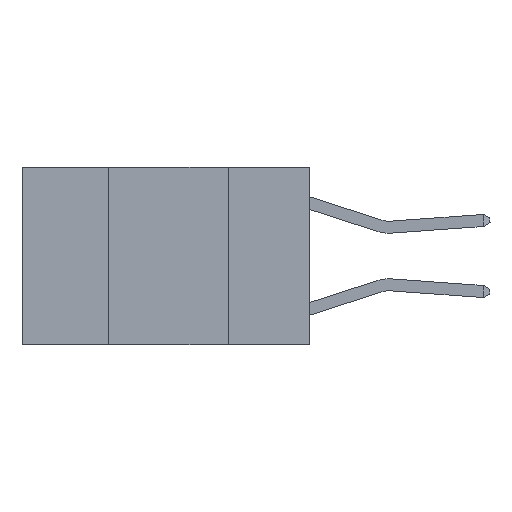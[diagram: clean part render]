
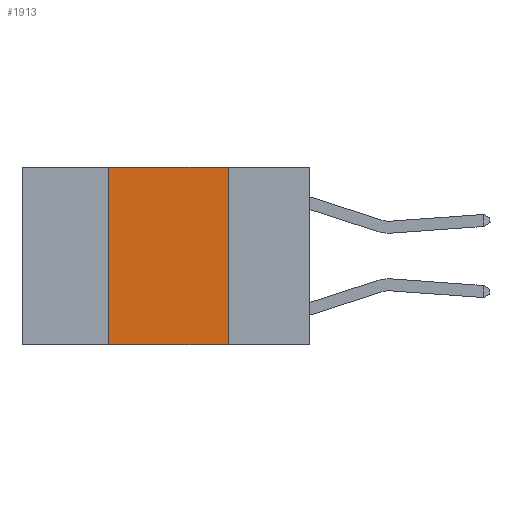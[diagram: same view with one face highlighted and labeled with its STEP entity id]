
A CAD part, left-side view. The second image highlights one B-rep face of the part: STEP entity #1913.
In plain terms, the highlighted planar face has unit normal (-1, 0, 0).
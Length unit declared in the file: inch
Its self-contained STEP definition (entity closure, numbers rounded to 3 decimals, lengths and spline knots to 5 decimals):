
#260 = VECTOR ( 'NONE', #7534, 39.37008 ) ;
#488 = CARTESIAN_POINT ( 'NONE',  ( 0., 0.17, -0.37 ) ) ;
#896 = CARTESIAN_POINT ( 'NONE',  ( 0., 0.6, -0.37 ) ) ;
#914 = LINE ( 'NONE', #11250, #3595 ) ;
#1346 = AXIS2_PLACEMENT_3D ( 'NONE', #8076, #11667, #6297 ) ;
#1599 = VERTEX_POINT ( 'NONE', #488 ) ;
#1626 = ORIENTED_EDGE ( 'NONE', *, *, #5721, .F. ) ;
#1913 = ADVANCED_FACE ( 'NONE', ( #11395 ), #10786, .F. ) ;
#2496 = CARTESIAN_POINT ( 'NONE',  ( 0., 0.6, 0. ) ) ;
#3595 = VECTOR ( 'NONE', #9520, 39.37008 ) ;
#3722 = VERTEX_POINT ( 'NONE', #9327 ) ;
#3993 = VERTEX_POINT ( 'NONE', #6340 ) ;
#4448 = VECTOR ( 'NONE', #7520, 39.37008 ) ;
#4730 = CARTESIAN_POINT ( 'NONE',  ( 0., 0.42, 0. ) ) ;
#4772 = LINE ( 'NONE', #2496, #11710 ) ;
#4922 = ORIENTED_EDGE ( 'NONE', *, *, #9820, .T. ) ;
#5017 = VERTEX_POINT ( 'NONE', #7310 ) ;
#5721 = EDGE_CURVE ( 'NONE', #5017, #3722, #4772, .T. ) ;
#6297 = DIRECTION ( 'NONE',  ( 0., 0., -1. ) ) ;
#6340 = CARTESIAN_POINT ( 'NONE',  ( 0., 0.42, -0.37 ) ) ;
#6675 = ORIENTED_EDGE ( 'NONE', *, *, #8371, .F. ) ;
#7098 = DIRECTION ( 'NONE',  ( 0., -1., 0. ) ) ;
#7310 = CARTESIAN_POINT ( 'NONE',  ( 0., 0.42, 0. ) ) ;
#7520 = DIRECTION ( 'NONE',  ( 0., 0., 1. ) ) ;
#7534 = DIRECTION ( 'NONE',  ( 0., -1., 0. ) ) ;
#8076 = CARTESIAN_POINT ( 'NONE',  ( 0., 0.6, 0. ) ) ;
#8241 = EDGE_CURVE ( 'NONE', #3993, #5017, #11684, .T. ) ;
#8371 = EDGE_CURVE ( 'NONE', #3722, #1599, #914, .T. ) ;
#9327 = CARTESIAN_POINT ( 'NONE',  ( 0., 0.17, 0. ) ) ;
#9520 = DIRECTION ( 'NONE',  ( 0., 0., -1. ) ) ;
#9717 = LINE ( 'NONE', #896, #260 ) ;
#9820 = EDGE_CURVE ( 'NONE', #3993, #1599, #9717, .T. ) ;
#10022 = ORIENTED_EDGE ( 'NONE', *, *, #8241, .F. ) ;
#10786 = PLANE ( 'NONE',  #1346 ) ;
#11250 = CARTESIAN_POINT ( 'NONE',  ( 0., 0.17, 0. ) ) ;
#11395 = FACE_OUTER_BOUND ( 'NONE', #11658, .T. ) ;
#11658 = EDGE_LOOP ( 'NONE', ( #6675, #1626, #10022, #4922 ) ) ;
#11667 = DIRECTION ( 'NONE',  ( 1., 0., 0. ) ) ;
#11684 = LINE ( 'NONE', #4730, #4448 ) ;
#11710 = VECTOR ( 'NONE', #7098, 39.37008 ) ;
